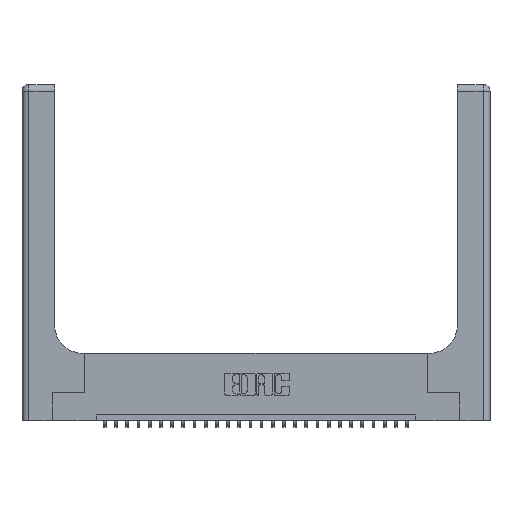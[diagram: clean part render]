
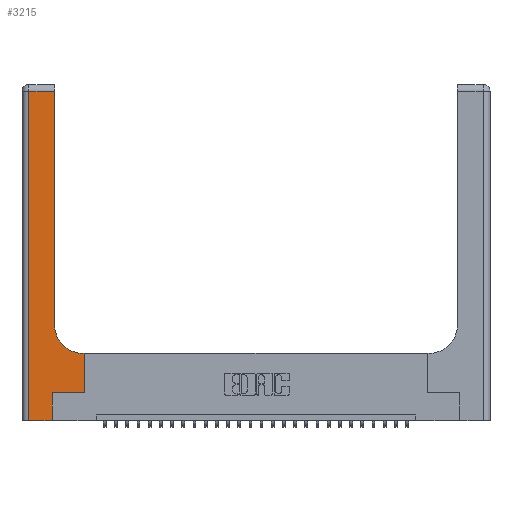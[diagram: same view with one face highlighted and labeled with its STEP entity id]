
A CAD part, top view. The second image highlights one B-rep face of the part: STEP entity #3215.
In plain terms, the highlighted planar face has unit normal (0, 0, 1).
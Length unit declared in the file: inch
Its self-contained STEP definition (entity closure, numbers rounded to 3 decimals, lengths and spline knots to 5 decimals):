
#259 = VECTOR ( 'NONE', #466, 39.37008 ) ;
#267 = DIRECTION ( 'NONE',  ( 0., 0., -1. ) ) ;
#466 = DIRECTION ( 'NONE',  ( 0., 1., 0. ) ) ;
#572 = ORIENTED_EDGE ( 'NONE', *, *, #24978, .T. ) ;
#820 = LINE ( 'NONE', #6667, #23306 ) ;
#2388 = FACE_OUTER_BOUND ( 'NONE', #10186, .T. ) ;
#2449 = AXIS2_PLACEMENT_3D ( 'NONE', #13287, #267, #15664 ) ;
#3215 = ADVANCED_FACE ( 'NONE', ( #2388 ), #21249, .F. ) ;
#3331 = EDGE_CURVE ( 'NONE', #11607, #12831, #27571, .T. ) ;
#4129 = VERTEX_POINT ( 'NONE', #15633 ) ;
#4240 = CARTESIAN_POINT ( 'NONE',  ( 0.2915, 3., 0.37 ) ) ;
#4487 = VERTEX_POINT ( 'NONE', #15107 ) ;
#4999 = CARTESIAN_POINT ( 'NONE',  ( 0.269, 0.25, 0.37 ) ) ;
#5068 = LINE ( 'NONE', #12790, #21742 ) ;
#6072 = ORIENTED_EDGE ( 'NONE', *, *, #27960, .T. ) ;
#6242 = DIRECTION ( 'NONE',  ( -1., 0., 0. ) ) ;
#6516 = LINE ( 'NONE', #16299, #19070 ) ;
#6667 = CARTESIAN_POINT ( 'NONE',  ( 0.06, 3., 0.37 ) ) ;
#6751 = LINE ( 'NONE', #22785, #259 ) ;
#7736 = DIRECTION ( 'NONE',  ( 0., 1., 0. ) ) ;
#8216 = DIRECTION ( 'NONE',  ( 0., 0., -1. ) ) ;
#8767 = VERTEX_POINT ( 'NONE', #14490 ) ;
#8838 = ORIENTED_EDGE ( 'NONE', *, *, #11893, .T. ) ;
#9927 = ORIENTED_EDGE ( 'NONE', *, *, #18757, .T. ) ;
#10186 = EDGE_LOOP ( 'NONE', ( #26042, #27438, #572, #9927, #17544, #10334, #6072, #8838, #19833 ) ) ;
#10323 = EDGE_CURVE ( 'NONE', #14515, #14977, #20362, .T. ) ;
#10334 = ORIENTED_EDGE ( 'NONE', *, *, #10323, .T. ) ;
#10517 = EDGE_CURVE ( 'NONE', #12831, #8767, #22387, .T. ) ;
#10691 = CARTESIAN_POINT ( 'NONE',  ( 0., 3., 0.37 ) ) ;
#11441 = CARTESIAN_POINT ( 'NONE',  ( 0.2915, 2.94, 0.37 ) ) ;
#11607 = VERTEX_POINT ( 'NONE', #18616 ) ;
#11704 = EDGE_CURVE ( 'NONE', #4487, #14515, #6751, .T. ) ;
#11893 = EDGE_CURVE ( 'NONE', #4129, #12694, #5068, .T. ) ;
#12607 = CARTESIAN_POINT ( 'NONE',  ( 0.269, 0.25, 0.37 ) ) ;
#12678 = CIRCLE ( 'NONE', #2449, 0.25 ) ;
#12694 = VERTEX_POINT ( 'NONE', #15888 ) ;
#12790 = CARTESIAN_POINT ( 'NONE',  ( 0.2915, 0.6, 0.37 ) ) ;
#12831 = VERTEX_POINT ( 'NONE', #11441 ) ;
#13287 = CARTESIAN_POINT ( 'NONE',  ( 0.5415, 0.85, 0.37 ) ) ;
#14490 = CARTESIAN_POINT ( 'NONE',  ( 0.06, 2.94, 0.37 ) ) ;
#14515 = VERTEX_POINT ( 'NONE', #12607 ) ;
#14558 = CARTESIAN_POINT ( 'NONE',  ( 0., 0., 0.37 ) ) ;
#14895 = VECTOR ( 'NONE', #27501, 39.37008 ) ;
#14977 = VERTEX_POINT ( 'NONE', #25316 ) ;
#15107 = CARTESIAN_POINT ( 'NONE',  ( 0.269, 0., 0.37 ) ) ;
#15633 = CARTESIAN_POINT ( 'NONE',  ( 0.5585, 0.6, 0.37 ) ) ;
#15664 = DIRECTION ( 'NONE',  ( 1., 0., 0. ) ) ;
#15888 = CARTESIAN_POINT ( 'NONE',  ( 0.5415, 0.6, 0.37 ) ) ;
#16299 = CARTESIAN_POINT ( 'NONE',  ( 0.5585, 0.25, 0.37 ) ) ;
#16688 = DIRECTION ( 'NONE',  ( -1., 0., 0. ) ) ;
#16865 = DIRECTION ( 'NONE',  ( 0., 1., 0. ) ) ;
#17544 = ORIENTED_EDGE ( 'NONE', *, *, #11704, .T. ) ;
#18490 = AXIS2_PLACEMENT_3D ( 'NONE', #10691, #8216, #6242 ) ;
#18616 = CARTESIAN_POINT ( 'NONE',  ( 0.2915, 0.85, 0.37 ) ) ;
#18644 = CARTESIAN_POINT ( 'NONE',  ( 0., 2.94, 0.37 ) ) ;
#18757 = EDGE_CURVE ( 'NONE', #25133, #4487, #22063, .T. ) ;
#19070 = VECTOR ( 'NONE', #7736, 39.37008 ) ;
#19833 = ORIENTED_EDGE ( 'NONE', *, *, #22711, .T. ) ;
#20270 = DIRECTION ( 'NONE',  ( 1., 0., 0. ) ) ;
#20362 = LINE ( 'NONE', #4999, #25126 ) ;
#20849 = DIRECTION ( 'NONE',  ( -1., 0., 0. ) ) ;
#21107 = VECTOR ( 'NONE', #16865, 39.37008 ) ;
#21249 = PLANE ( 'NONE',  #18490 ) ;
#21742 = VECTOR ( 'NONE', #16688, 39.37008 ) ;
#22063 = LINE ( 'NONE', #14558, #14895 ) ;
#22387 = LINE ( 'NONE', #18644, #23427 ) ;
#22711 = EDGE_CURVE ( 'NONE', #12694, #11607, #12678, .T. ) ;
#22785 = CARTESIAN_POINT ( 'NONE',  ( 0.269, 0., 0.37 ) ) ;
#23306 = VECTOR ( 'NONE', #24046, 39.37008 ) ;
#23427 = VECTOR ( 'NONE', #20849, 39.37008 ) ;
#24046 = DIRECTION ( 'NONE',  ( 0., -1., 0. ) ) ;
#24978 = EDGE_CURVE ( 'NONE', #8767, #25133, #820, .T. ) ;
#25126 = VECTOR ( 'NONE', #20270, 39.37008 ) ;
#25133 = VERTEX_POINT ( 'NONE', #26610 ) ;
#25316 = CARTESIAN_POINT ( 'NONE',  ( 0.5585, 0.25, 0.37 ) ) ;
#26042 = ORIENTED_EDGE ( 'NONE', *, *, #3331, .T. ) ;
#26610 = CARTESIAN_POINT ( 'NONE',  ( 0.06, 0., 0.37 ) ) ;
#27438 = ORIENTED_EDGE ( 'NONE', *, *, #10517, .T. ) ;
#27501 = DIRECTION ( 'NONE',  ( 1., 0., 0. ) ) ;
#27571 = LINE ( 'NONE', #4240, #21107 ) ;
#27960 = EDGE_CURVE ( 'NONE', #14977, #4129, #6516, .T. ) ;
